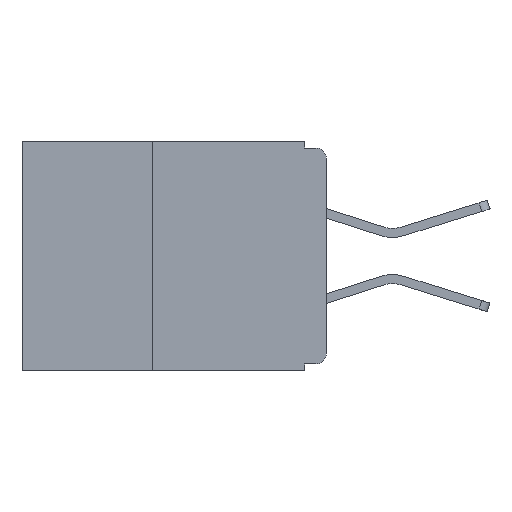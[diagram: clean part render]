
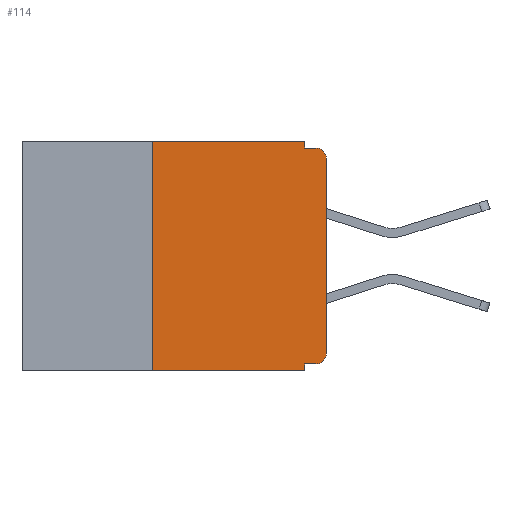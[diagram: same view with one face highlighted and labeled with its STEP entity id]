
A CAD part, left-side view. The second image highlights one B-rep face of the part: STEP entity #114.
In plain terms, the highlighted planar face has unit normal (-1, 0, 0).
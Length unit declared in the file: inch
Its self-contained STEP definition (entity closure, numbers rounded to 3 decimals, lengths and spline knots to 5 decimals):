
#114 = ADVANCED_FACE ( 'NONE', ( #12934 ), #2627, .F. ) ;
#139 = CARTESIAN_POINT ( 'NONE',  ( 0., 0.031, -0.33 ) ) ;
#191 = DIRECTION ( 'NONE',  ( 0., -1., 0. ) ) ;
#206 = VECTOR ( 'NONE', #21600, 39.37008 ) ;
#446 = ORIENTED_EDGE ( 'NONE', *, *, #19530, .T. ) ;
#733 = LINE ( 'NONE', #7138, #5286 ) ;
#1464 = DIRECTION ( 'NONE',  ( 1., 0., 0. ) ) ;
#1513 = VERTEX_POINT ( 'NONE', #2566 ) ;
#1959 = EDGE_CURVE ( 'NONE', #18350, #15434, #2412, .T. ) ;
#2412 = LINE ( 'NONE', #23491, #12222 ) ;
#2566 = CARTESIAN_POINT ( 'NONE',  ( 0., 0.031, -0.32 ) ) ;
#2575 = VERTEX_POINT ( 'NONE', #18308 ) ;
#2627 = PLANE ( 'NONE',  #5873 ) ;
#2808 = CARTESIAN_POINT ( 'NONE',  ( 0., 0., -0.01 ) ) ;
#3087 = EDGE_CURVE ( 'NONE', #19619, #9906, #16750, .T. ) ;
#3520 = ORIENTED_EDGE ( 'NONE', *, *, #3087, .F. ) ;
#3580 = DIRECTION ( 'NONE',  ( 0., -1., 0. ) ) ;
#3849 = EDGE_CURVE ( 'NONE', #2575, #1513, #15808, .T. ) ;
#4165 = CARTESIAN_POINT ( 'NONE',  ( 0., 0.031, 0. ) ) ;
#4542 = EDGE_CURVE ( 'NONE', #9906, #10538, #18685, .T. ) ;
#4650 = LINE ( 'NONE', #23469, #13844 ) ;
#5286 = VECTOR ( 'NONE', #7076, 39.37008 ) ;
#5292 = CIRCLE ( 'NONE', #5618, 0.015 ) ;
#5428 = DIRECTION ( 'NONE',  ( 0., 0., -1. ) ) ;
#5470 = CARTESIAN_POINT ( 'NONE',  ( 0., 0.031, -0.01 ) ) ;
#5618 = AXIS2_PLACEMENT_3D ( 'NONE', #22674, #11090, #24565 ) ;
#5705 = VECTOR ( 'NONE', #5428, 39.37008 ) ;
#5709 = DIRECTION ( 'NONE',  ( -1., 0., 0. ) ) ;
#5873 = AXIS2_PLACEMENT_3D ( 'NONE', #12125, #1464, #6180 ) ;
#6180 = DIRECTION ( 'NONE',  ( 0., 0., -1. ) ) ;
#6809 = CARTESIAN_POINT ( 'NONE',  ( 0., 0., -0.025 ) ) ;
#7076 = DIRECTION ( 'NONE',  ( 0., -1., 0. ) ) ;
#7138 = CARTESIAN_POINT ( 'NONE',  ( 0., 0.437, 0. ) ) ;
#7182 = ORIENTED_EDGE ( 'NONE', *, *, #13956, .F. ) ;
#8044 = CARTESIAN_POINT ( 'NONE',  ( 0., 0.031, 0. ) ) ;
#8321 = VECTOR ( 'NONE', #3580, 39.37008 ) ;
#8608 = AXIS2_PLACEMENT_3D ( 'NONE', #17425, #5709, #19369 ) ;
#9483 = EDGE_CURVE ( 'NONE', #17488, #9785, #21160, .T. ) ;
#9785 = VERTEX_POINT ( 'NONE', #6809 ) ;
#9906 = VERTEX_POINT ( 'NONE', #5470 ) ;
#10155 = CARTESIAN_POINT ( 'NONE',  ( 0., 0., 0. ) ) ;
#10232 = ORIENTED_EDGE ( 'NONE', *, *, #9483, .T. ) ;
#10240 = DIRECTION ( 'NONE',  ( 0., 0., 1. ) ) ;
#10538 = VERTEX_POINT ( 'NONE', #14310 ) ;
#10658 = EDGE_CURVE ( 'NONE', #15434, #19619, #733, .T. ) ;
#11090 = DIRECTION ( 'NONE',  ( -1., 0., 0. ) ) ;
#12125 = CARTESIAN_POINT ( 'NONE',  ( 0., 0.437, 0. ) ) ;
#12222 = VECTOR ( 'NONE', #18509, 39.37008 ) ;
#12859 = VECTOR ( 'NONE', #20121, 39.37008 ) ;
#12934 = FACE_OUTER_BOUND ( 'NONE', #21141, .T. ) ;
#13322 = ORIENTED_EDGE ( 'NONE', *, *, #4542, .F. ) ;
#13844 = VECTOR ( 'NONE', #191, 39.37008 ) ;
#13956 = EDGE_CURVE ( 'NONE', #1513, #17450, #23701, .T. ) ;
#14257 = ORIENTED_EDGE ( 'NONE', *, *, #18609, .T. ) ;
#14310 = CARTESIAN_POINT ( 'NONE',  ( 0., 0.015, -0.01 ) ) ;
#15434 = VERTEX_POINT ( 'NONE', #20836 ) ;
#15685 = CIRCLE ( 'NONE', #8608, 0.015 ) ;
#15759 = ORIENTED_EDGE ( 'NONE', *, *, #10658, .F. ) ;
#15808 = LINE ( 'NONE', #21656, #206 ) ;
#15867 = CARTESIAN_POINT ( 'NONE',  ( 0., 0., -0.305 ) ) ;
#16072 = CARTESIAN_POINT ( 'NONE',  ( 0., 0.25, -0.33 ) ) ;
#16750 = LINE ( 'NONE', #4165, #5705 ) ;
#16968 = ORIENTED_EDGE ( 'NONE', *, *, #19601, .T. ) ;
#17425 = CARTESIAN_POINT ( 'NONE',  ( 0., 0.015, -0.025 ) ) ;
#17450 = VERTEX_POINT ( 'NONE', #139 ) ;
#17488 = VERTEX_POINT ( 'NONE', #15867 ) ;
#18161 = CARTESIAN_POINT ( 'NONE',  ( 0., 0.031, -0.33 ) ) ;
#18166 = ORIENTED_EDGE ( 'NONE', *, *, #3849, .F. ) ;
#18308 = CARTESIAN_POINT ( 'NONE',  ( 0., 0.015, -0.32 ) ) ;
#18350 = VERTEX_POINT ( 'NONE', #16072 ) ;
#18509 = DIRECTION ( 'NONE',  ( 0., 0., 1. ) ) ;
#18609 = EDGE_CURVE ( 'NONE', #2575, #17488, #5292, .T. ) ;
#18685 = LINE ( 'NONE', #2808, #8321 ) ;
#19369 = DIRECTION ( 'NONE',  ( 0., 0., -1. ) ) ;
#19530 = EDGE_CURVE ( 'NONE', #9785, #10538, #15685, .T. ) ;
#19601 = EDGE_CURVE ( 'NONE', #18350, #17450, #4650, .T. ) ;
#19619 = VERTEX_POINT ( 'NONE', #8044 ) ;
#20121 = DIRECTION ( 'NONE',  ( 0., 0., -1. ) ) ;
#20564 = VECTOR ( 'NONE', #10240, 39.37008 ) ;
#20836 = CARTESIAN_POINT ( 'NONE',  ( 0., 0.25, 0. ) ) ;
#20878 = ORIENTED_EDGE ( 'NONE', *, *, #1959, .F. ) ;
#21141 = EDGE_LOOP ( 'NONE', ( #10232, #446, #13322, #3520, #15759, #20878, #16968, #7182, #18166, #14257 ) ) ;
#21160 = LINE ( 'NONE', #10155, #20564 ) ;
#21600 = DIRECTION ( 'NONE',  ( 0., 1., 0. ) ) ;
#21656 = CARTESIAN_POINT ( 'NONE',  ( 0., 0., -0.32 ) ) ;
#22674 = CARTESIAN_POINT ( 'NONE',  ( 0., 0.015, -0.305 ) ) ;
#23469 = CARTESIAN_POINT ( 'NONE',  ( 0., 0.437, -0.33 ) ) ;
#23491 = CARTESIAN_POINT ( 'NONE',  ( 0., 0.25, -0.33 ) ) ;
#23701 = LINE ( 'NONE', #18161, #12859 ) ;
#24565 = DIRECTION ( 'NONE',  ( 0., 0., -1. ) ) ;
